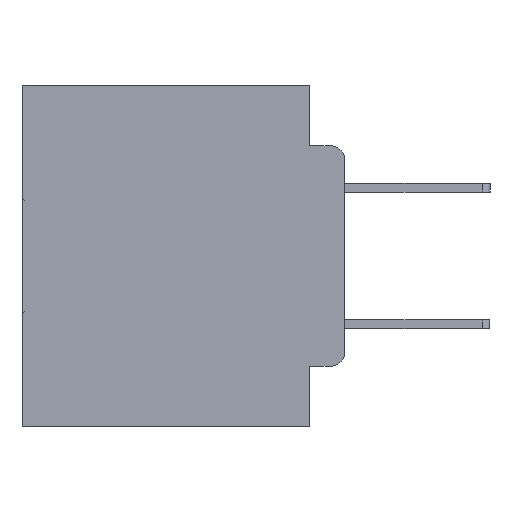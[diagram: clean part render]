
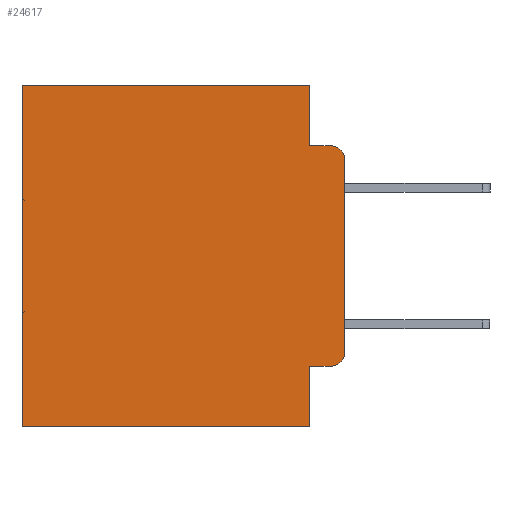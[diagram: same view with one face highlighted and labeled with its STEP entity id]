
A CAD part, left-side view. The second image highlights one B-rep face of the part: STEP entity #24617.
In plain terms, the highlighted planar face has unit normal (-1, 0, 0).
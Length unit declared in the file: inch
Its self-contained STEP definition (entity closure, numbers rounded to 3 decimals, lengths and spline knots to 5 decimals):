
#94 = CARTESIAN_POINT ( 'NONE',  ( 0.298, 0., -0.1085 ) ) ;
#455 = LINE ( 'NONE', #26416, #19651 ) ;
#481 = EDGE_LOOP ( 'NONE', ( #25775, #10320, #19513, #14355, #6982, #19496, #2582, #22576, #26851, #28201 ) ) ;
#827 = VERTEX_POINT ( 'NONE', #94 ) ;
#1891 = LINE ( 'NONE', #6780, #13701 ) ;
#2403 = EDGE_CURVE ( 'NONE', #23399, #28618, #31111, .T. ) ;
#2582 = ORIENTED_EDGE ( 'NONE', *, *, #5450, .F. ) ;
#2828 = VERTEX_POINT ( 'NONE', #3476 ) ;
#3476 = CARTESIAN_POINT ( 'NONE',  ( 0.298, 0.02, -0.4115 ) ) ;
#4811 = VECTOR ( 'NONE', #27144, 39.37008 ) ;
#5450 = EDGE_CURVE ( 'NONE', #10339, #25272, #30222, .T. ) ;
#5484 = CARTESIAN_POINT ( 'NONE',  ( 0.298, 0.051, -0.5 ) ) ;
#5502 = CARTESIAN_POINT ( 'NONE',  ( 0.298, 0.051, -0.0885 ) ) ;
#6046 = DIRECTION ( 'NONE',  ( 1., 0., 0. ) ) ;
#6493 = FACE_OUTER_BOUND ( 'NONE', #481, .T. ) ;
#6568 = CARTESIAN_POINT ( 'NONE',  ( 0.298, 0.473, 0. ) ) ;
#6780 = CARTESIAN_POINT ( 'NONE',  ( 0.298, 0., 0. ) ) ;
#6845 = CARTESIAN_POINT ( 'NONE',  ( 0.298, 0., 0. ) ) ;
#6982 = ORIENTED_EDGE ( 'NONE', *, *, #2403, .T. ) ;
#8679 = DIRECTION ( 'NONE',  ( 0., 0., -1. ) ) ;
#10031 = LINE ( 'NONE', #28129, #29563 ) ;
#10320 = ORIENTED_EDGE ( 'NONE', *, *, #23802, .T. ) ;
#10332 = VECTOR ( 'NONE', #31359, 39.37008 ) ;
#10339 = VERTEX_POINT ( 'NONE', #5484 ) ;
#10624 = EDGE_CURVE ( 'NONE', #11618, #2828, #455, .T. ) ;
#10869 = VECTOR ( 'NONE', #19219, 39.37008 ) ;
#10922 = CIRCLE ( 'NONE', #16376, 0.02 ) ;
#11493 = EDGE_CURVE ( 'NONE', #2828, #22143, #10922, .T. ) ;
#11618 = VERTEX_POINT ( 'NONE', #11662 ) ;
#11662 = CARTESIAN_POINT ( 'NONE',  ( 0.298, 0.051, -0.4115 ) ) ;
#12391 = LINE ( 'NONE', #23469, #25429 ) ;
#12448 = CARTESIAN_POINT ( 'NONE',  ( 0.298, 0., -0.5 ) ) ;
#12684 = DIRECTION ( 'NONE',  ( -1., 0., 0. ) ) ;
#13480 = DIRECTION ( 'NONE',  ( 0., 0., -1. ) ) ;
#13507 = CARTESIAN_POINT ( 'NONE',  ( 0.298, 0., 0. ) ) ;
#13701 = VECTOR ( 'NONE', #21621, 39.37008 ) ;
#13732 = CARTESIAN_POINT ( 'NONE',  ( 0.298, 0.02, -0.3915 ) ) ;
#13953 = EDGE_CURVE ( 'NONE', #11618, #10339, #10031, .T. ) ;
#14355 = ORIENTED_EDGE ( 'NONE', *, *, #18881, .F. ) ;
#14434 = CARTESIAN_POINT ( 'NONE',  ( 0.298, 0.473, 0. ) ) ;
#14576 = LINE ( 'NONE', #14434, #20325 ) ;
#15607 = EDGE_CURVE ( 'NONE', #28618, #25272, #14576, .T. ) ;
#15943 = CARTESIAN_POINT ( 'NONE',  ( 0.298, 0.473, -0.5 ) ) ;
#16188 = DIRECTION ( 'NONE',  ( 0., 0., -1. ) ) ;
#16376 = AXIS2_PLACEMENT_3D ( 'NONE', #13732, #30754, #16188 ) ;
#16418 = AXIS2_PLACEMENT_3D ( 'NONE', #27360, #12684, #29762 ) ;
#18222 = CARTESIAN_POINT ( 'NONE',  ( 0.298, 0., -0.3915 ) ) ;
#18268 = CIRCLE ( 'NONE', #16418, 0.02 ) ;
#18881 = EDGE_CURVE ( 'NONE', #23399, #24475, #12391, .T. ) ;
#19219 = DIRECTION ( 'NONE',  ( 0., 1., 0. ) ) ;
#19496 = ORIENTED_EDGE ( 'NONE', *, *, #15607, .T. ) ;
#19513 = ORIENTED_EDGE ( 'NONE', *, *, #20525, .F. ) ;
#19651 = VECTOR ( 'NONE', #31244, 39.37008 ) ;
#20325 = VECTOR ( 'NONE', #29061, 39.37008 ) ;
#20525 = EDGE_CURVE ( 'NONE', #24475, #27858, #30579, .T. ) ;
#20912 = PLANE ( 'NONE',  #31505 ) ;
#21621 = DIRECTION ( 'NONE',  ( 0., 0., -1. ) ) ;
#22143 = VERTEX_POINT ( 'NONE', #18222 ) ;
#22576 = ORIENTED_EDGE ( 'NONE', *, *, #13953, .F. ) ;
#23371 = DIRECTION ( 'NONE',  ( 0., 0., -1. ) ) ;
#23399 = VERTEX_POINT ( 'NONE', #28110 ) ;
#23469 = CARTESIAN_POINT ( 'NONE',  ( 0.298, 0.051, 0. ) ) ;
#23802 = EDGE_CURVE ( 'NONE', #827, #27858, #18268, .T. ) ;
#24084 = CARTESIAN_POINT ( 'NONE',  ( 0.298, 0.051, -0.0885 ) ) ;
#24475 = VERTEX_POINT ( 'NONE', #5502 ) ;
#24617 = ADVANCED_FACE ( 'NONE', ( #6493 ), #20912, .F. ) ;
#25272 = VERTEX_POINT ( 'NONE', #15943 ) ;
#25285 = CARTESIAN_POINT ( 'NONE',  ( 0.298, 0.02, -0.0885 ) ) ;
#25429 = VECTOR ( 'NONE', #8679, 39.37008 ) ;
#25775 = ORIENTED_EDGE ( 'NONE', *, *, #28679, .F. ) ;
#26416 = CARTESIAN_POINT ( 'NONE',  ( 0.298, 0.051, -0.4115 ) ) ;
#26851 = ORIENTED_EDGE ( 'NONE', *, *, #10624, .T. ) ;
#27144 = DIRECTION ( 'NONE',  ( 0., 1., 0. ) ) ;
#27360 = CARTESIAN_POINT ( 'NONE',  ( 0.298, 0.02, -0.1085 ) ) ;
#27858 = VERTEX_POINT ( 'NONE', #25285 ) ;
#28110 = CARTESIAN_POINT ( 'NONE',  ( 0.298, 0.051, 0. ) ) ;
#28129 = CARTESIAN_POINT ( 'NONE',  ( 0.298, 0.051, 0. ) ) ;
#28201 = ORIENTED_EDGE ( 'NONE', *, *, #11493, .T. ) ;
#28618 = VERTEX_POINT ( 'NONE', #6568 ) ;
#28679 = EDGE_CURVE ( 'NONE', #827, #22143, #1891, .T. ) ;
#29061 = DIRECTION ( 'NONE',  ( 0., 0., -1. ) ) ;
#29563 = VECTOR ( 'NONE', #13480, 39.37008 ) ;
#29762 = DIRECTION ( 'NONE',  ( 0., 0., -1. ) ) ;
#30222 = LINE ( 'NONE', #12448, #4811 ) ;
#30579 = LINE ( 'NONE', #24084, #10332 ) ;
#30754 = DIRECTION ( 'NONE',  ( -1., 0., 0. ) ) ;
#31111 = LINE ( 'NONE', #6845, #10869 ) ;
#31244 = DIRECTION ( 'NONE',  ( 0., -1., 0. ) ) ;
#31359 = DIRECTION ( 'NONE',  ( 0., -1., 0. ) ) ;
#31505 = AXIS2_PLACEMENT_3D ( 'NONE', #13507, #6046, #23371 ) ;
